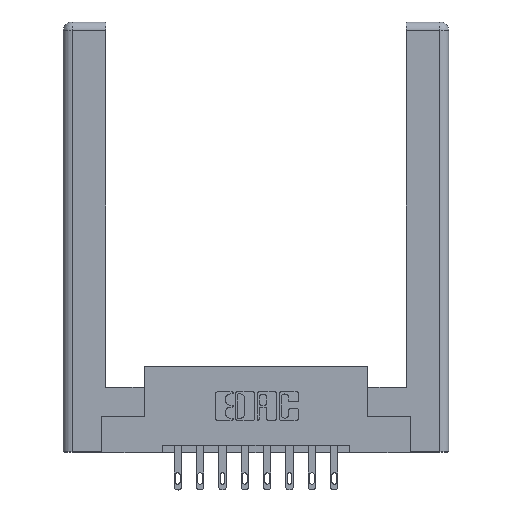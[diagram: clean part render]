
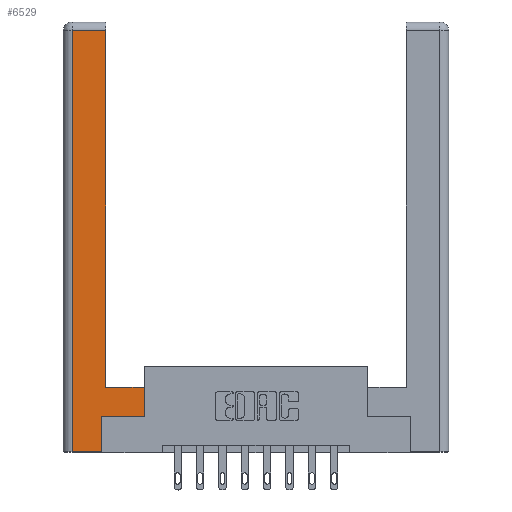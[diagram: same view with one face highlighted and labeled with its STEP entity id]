
A CAD part, top view. The second image highlights one B-rep face of the part: STEP entity #6529.
In plain terms, the highlighted planar face has unit normal (0, 0, 1).
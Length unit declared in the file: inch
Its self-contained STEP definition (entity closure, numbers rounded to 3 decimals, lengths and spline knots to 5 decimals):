
#1 = EDGE_CURVE ( 'NONE', #11268, #2606, #10053, .T. ) ;
#311 = DIRECTION ( 'NONE',  ( 0., -1., 0. ) ) ;
#608 = VECTOR ( 'NONE', #10248, 39.37008 ) ;
#995 = CARTESIAN_POINT ( 'NONE',  ( 0.565, 0.45, 0. ) ) ;
#1424 = VECTOR ( 'NONE', #311, 39.37008 ) ;
#1628 = ORIENTED_EDGE ( 'NONE', *, *, #2630, .T. ) ;
#1655 = VERTEX_POINT ( 'NONE', #7566 ) ;
#2333 = ORIENTED_EDGE ( 'NONE', *, *, #5362, .T. ) ;
#2381 = CARTESIAN_POINT ( 'NONE',  ( 0.265, 0.245, 0. ) ) ;
#2606 = VERTEX_POINT ( 'NONE', #9144 ) ;
#2630 = EDGE_CURVE ( 'NONE', #12479, #13137, #4879, .T. ) ;
#2776 = EDGE_CURVE ( 'NONE', #11584, #12479, #5992, .T. ) ;
#2842 = LINE ( 'NONE', #11609, #1424 ) ;
#3110 = CARTESIAN_POINT ( 'NONE',  ( 0.295, 2.94, 0. ) ) ;
#3363 = DIRECTION ( 'NONE',  ( 0., 1., 0. ) ) ;
#3564 = DIRECTION ( 'NONE',  ( 0., 0., -1. ) ) ;
#3714 = LINE ( 'NONE', #2381, #11517 ) ;
#3844 = ORIENTED_EDGE ( 'NONE', *, *, #5895, .T. ) ;
#4230 = FACE_OUTER_BOUND ( 'NONE', #6570, .T. ) ;
#4333 = ORIENTED_EDGE ( 'NONE', *, *, #2776, .T. ) ;
#4476 = EDGE_CURVE ( 'NONE', #7859, #11268, #2842, .T. ) ;
#4579 = LINE ( 'NONE', #8634, #12680 ) ;
#4818 = ORIENTED_EDGE ( 'NONE', *, *, #6358, .T. ) ;
#4879 = LINE ( 'NONE', #995, #608 ) ;
#5362 = EDGE_CURVE ( 'NONE', #1655, #5473, #8080, .T. ) ;
#5473 = VERTEX_POINT ( 'NONE', #3110 ) ;
#5639 = PLANE ( 'NONE',  #5677 ) ;
#5677 = AXIS2_PLACEMENT_3D ( 'NONE', #8625, #3564, #12607 ) ;
#5895 = EDGE_CURVE ( 'NONE', #5473, #7859, #4579, .T. ) ;
#5992 = LINE ( 'NONE', #11445, #8401 ) ;
#6328 = CARTESIAN_POINT ( 'NONE',  ( 0.295, 3., 0. ) ) ;
#6358 = EDGE_CURVE ( 'NONE', #13137, #1655, #9182, .T. ) ;
#6432 = ORIENTED_EDGE ( 'NONE', *, *, #11648, .T. ) ;
#6471 = CARTESIAN_POINT ( 'NONE',  ( 0.565, 0.245, 0. ) ) ;
#6529 = ADVANCED_FACE ( 'NONE', ( #4230 ), #5639, .F. ) ;
#6570 = EDGE_LOOP ( 'NONE', ( #2333, #3844, #11966, #9764, #6432, #4333, #1628, #4818 ) ) ;
#6710 = DIRECTION ( 'NONE',  ( -1., 0., 0. ) ) ;
#6931 = DIRECTION ( 'NONE',  ( -1., 0., 0. ) ) ;
#7521 = CARTESIAN_POINT ( 'NONE',  ( 0.295, 0.45, 0. ) ) ;
#7566 = CARTESIAN_POINT ( 'NONE',  ( 0.295, 0.45, 0. ) ) ;
#7711 = CARTESIAN_POINT ( 'NONE',  ( 0.565, 0.45, 0. ) ) ;
#7859 = VERTEX_POINT ( 'NONE', #10699 ) ;
#8080 = LINE ( 'NONE', #6328, #13173 ) ;
#8401 = VECTOR ( 'NONE', #11394, 39.37008 ) ;
#8625 = CARTESIAN_POINT ( 'NONE',  ( 0., 0., 0. ) ) ;
#8634 = CARTESIAN_POINT ( 'NONE',  ( 0.0615, 2.94, 0. ) ) ;
#9144 = CARTESIAN_POINT ( 'NONE',  ( 0.265, 0., 0. ) ) ;
#9159 = CARTESIAN_POINT ( 'NONE',  ( 0.265, 0., 0. ) ) ;
#9182 = LINE ( 'NONE', #7521, #10781 ) ;
#9309 = CARTESIAN_POINT ( 'NONE',  ( 0.265, 0.245, 0. ) ) ;
#9605 = VECTOR ( 'NONE', #10094, 39.37008 ) ;
#9764 = ORIENTED_EDGE ( 'NONE', *, *, #1, .T. ) ;
#10053 = LINE ( 'NONE', #9159, #9605 ) ;
#10094 = DIRECTION ( 'NONE',  ( 1., 0., 0. ) ) ;
#10248 = DIRECTION ( 'NONE',  ( 0., 1., 0. ) ) ;
#10389 = DIRECTION ( 'NONE',  ( 0., 1., 0. ) ) ;
#10699 = CARTESIAN_POINT ( 'NONE',  ( 0.0615, 2.94, 0. ) ) ;
#10781 = VECTOR ( 'NONE', #6710, 39.37008 ) ;
#11268 = VERTEX_POINT ( 'NONE', #11839 ) ;
#11394 = DIRECTION ( 'NONE',  ( 1., 0., 0. ) ) ;
#11445 = CARTESIAN_POINT ( 'NONE',  ( 0.565, 0.245, 0. ) ) ;
#11517 = VECTOR ( 'NONE', #3363, 39.37008 ) ;
#11584 = VERTEX_POINT ( 'NONE', #9309 ) ;
#11609 = CARTESIAN_POINT ( 'NONE',  ( 0.0615, 0., 0. ) ) ;
#11648 = EDGE_CURVE ( 'NONE', #2606, #11584, #3714, .T. ) ;
#11839 = CARTESIAN_POINT ( 'NONE',  ( 0.0615, 0., 0. ) ) ;
#11966 = ORIENTED_EDGE ( 'NONE', *, *, #4476, .T. ) ;
#12479 = VERTEX_POINT ( 'NONE', #6471 ) ;
#12607 = DIRECTION ( 'NONE',  ( -1., 0., 0. ) ) ;
#12680 = VECTOR ( 'NONE', #6931, 39.37008 ) ;
#13137 = VERTEX_POINT ( 'NONE', #7711 ) ;
#13173 = VECTOR ( 'NONE', #10389, 39.37008 ) ;
